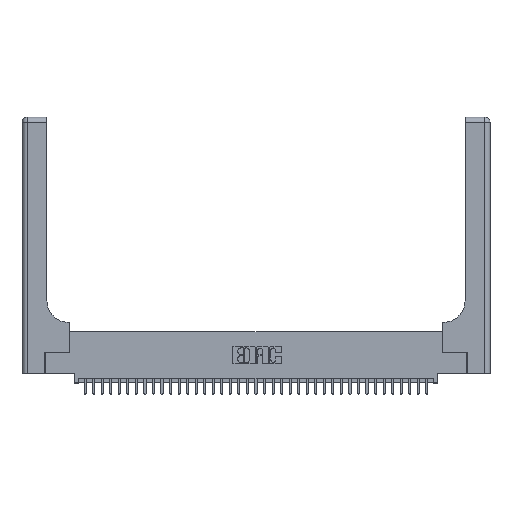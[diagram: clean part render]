
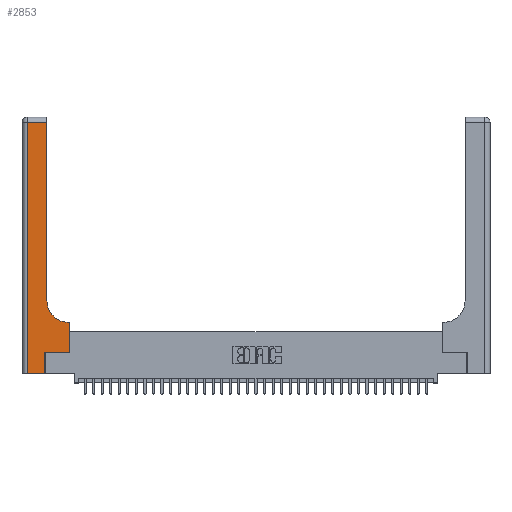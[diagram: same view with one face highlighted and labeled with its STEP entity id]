
A CAD part, top view. The second image highlights one B-rep face of the part: STEP entity #2853.
In plain terms, the highlighted planar face has unit normal (0, 0, 1).
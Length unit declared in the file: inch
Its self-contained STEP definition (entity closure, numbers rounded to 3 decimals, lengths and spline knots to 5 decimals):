
#905 = CARTESIAN_POINT ( 'NONE',  ( 0.269, 0., 0.37 ) ) ;
#2795 = VECTOR ( 'NONE', #10606, 39.37008 ) ;
#2853 = ADVANCED_FACE ( 'NONE', ( #34751 ), #29585, .F. ) ;
#3698 = VECTOR ( 'NONE', #23925, 39.37008 ) ;
#4071 = EDGE_CURVE ( 'NONE', #8317, #31394, #30599, .T. ) ;
#4381 = CARTESIAN_POINT ( 'NONE',  ( 0.269, 0.25, 0.37 ) ) ;
#4524 = DIRECTION ( 'NONE',  ( 1., 0., 0. ) ) ;
#4832 = CARTESIAN_POINT ( 'NONE',  ( 0.2915, 0.6, 0.37 ) ) ;
#5207 = DIRECTION ( 'NONE',  ( -1., 0., 0. ) ) ;
#5874 = EDGE_CURVE ( 'NONE', #9126, #23208, #30450, .T. ) ;
#6707 = ORIENTED_EDGE ( 'NONE', *, *, #24233, .T. ) ;
#7467 = VERTEX_POINT ( 'NONE', #4381 ) ;
#8197 = CARTESIAN_POINT ( 'NONE',  ( 0.2915, 2.94, 0.37 ) ) ;
#8317 = VERTEX_POINT ( 'NONE', #22243 ) ;
#9126 = VERTEX_POINT ( 'NONE', #8197 ) ;
#9229 = CARTESIAN_POINT ( 'NONE',  ( 0.269, 0., 0.37 ) ) ;
#10606 = DIRECTION ( 'NONE',  ( 0., 1., 0. ) ) ;
#10886 = CARTESIAN_POINT ( 'NONE',  ( 0.5415, 0.85, 0.37 ) ) ;
#11443 = VERTEX_POINT ( 'NONE', #30792 ) ;
#11769 = DIRECTION ( 'NONE',  ( 0., 0., -1. ) ) ;
#12270 = CARTESIAN_POINT ( 'NONE',  ( 0., 3., 0.37 ) ) ;
#12569 = ORIENTED_EDGE ( 'NONE', *, *, #26493, .T. ) ;
#13394 = CARTESIAN_POINT ( 'NONE',  ( 0.5585, 0.25, 0.37 ) ) ;
#13497 = EDGE_CURVE ( 'NONE', #31394, #7467, #32651, .T. ) ;
#14502 = DIRECTION ( 'NONE',  ( 0., -1., 0. ) ) ;
#15066 = DIRECTION ( 'NONE',  ( 0., 1., 0. ) ) ;
#16589 = LINE ( 'NONE', #25173, #21145 ) ;
#17792 = VERTEX_POINT ( 'NONE', #24611 ) ;
#18271 = EDGE_CURVE ( 'NONE', #7467, #28754, #29657, .T. ) ;
#18658 = EDGE_LOOP ( 'NONE', ( #36501, #22515, #12569, #22417, #20735, #31339, #27464, #6707, #30149 ) ) ;
#20735 = ORIENTED_EDGE ( 'NONE', *, *, #13497, .T. ) ;
#21145 = VECTOR ( 'NONE', #30897, 39.37008 ) ;
#21361 = CARTESIAN_POINT ( 'NONE',  ( 0.269, 0.25, 0.37 ) ) ;
#22243 = CARTESIAN_POINT ( 'NONE',  ( 0.06, 0., 0.37 ) ) ;
#22417 = ORIENTED_EDGE ( 'NONE', *, *, #4071, .T. ) ;
#22515 = ORIENTED_EDGE ( 'NONE', *, *, #5874, .T. ) ;
#23208 = VERTEX_POINT ( 'NONE', #29450 ) ;
#23925 = DIRECTION ( 'NONE',  ( 1., 0., 0. ) ) ;
#24233 = EDGE_CURVE ( 'NONE', #17792, #11443, #32466, .T. ) ;
#24611 = CARTESIAN_POINT ( 'NONE',  ( 0.5585, 0.6, 0.37 ) ) ;
#24971 = VECTOR ( 'NONE', #35437, 39.37008 ) ;
#25109 = AXIS2_PLACEMENT_3D ( 'NONE', #12270, #11769, #26641 ) ;
#25173 = CARTESIAN_POINT ( 'NONE',  ( 0.2915, 3., 0.37 ) ) ;
#25206 = CARTESIAN_POINT ( 'NONE',  ( 0.5585, 0.25, 0.37 ) ) ;
#25261 = EDGE_CURVE ( 'NONE', #28754, #17792, #32436, .T. ) ;
#26493 = EDGE_CURVE ( 'NONE', #23208, #8317, #37329, .T. ) ;
#26641 = DIRECTION ( 'NONE',  ( -1., 0., 0. ) ) ;
#27053 = VERTEX_POINT ( 'NONE', #28631 ) ;
#27394 = EDGE_CURVE ( 'NONE', #27053, #9126, #16589, .T. ) ;
#27464 = ORIENTED_EDGE ( 'NONE', *, *, #25261, .T. ) ;
#28631 = CARTESIAN_POINT ( 'NONE',  ( 0.2915, 0.85, 0.37 ) ) ;
#28754 = VERTEX_POINT ( 'NONE', #25206 ) ;
#29450 = CARTESIAN_POINT ( 'NONE',  ( 0.06, 2.94, 0.37 ) ) ;
#29585 = PLANE ( 'NONE',  #25109 ) ;
#29657 = LINE ( 'NONE', #21361, #3698 ) ;
#29946 = VECTOR ( 'NONE', #15066, 39.37008 ) ;
#29999 = CARTESIAN_POINT ( 'NONE',  ( 0., 2.94, 0.37 ) ) ;
#30149 = ORIENTED_EDGE ( 'NONE', *, *, #33298, .T. ) ;
#30450 = LINE ( 'NONE', #29999, #24971 ) ;
#30599 = LINE ( 'NONE', #35593, #31072 ) ;
#30777 = CIRCLE ( 'NONE', #31542, 0.25 ) ;
#30792 = CARTESIAN_POINT ( 'NONE',  ( 0.5415, 0.6, 0.37 ) ) ;
#30897 = DIRECTION ( 'NONE',  ( 0., 1., 0. ) ) ;
#31072 = VECTOR ( 'NONE', #35463, 39.37008 ) ;
#31339 = ORIENTED_EDGE ( 'NONE', *, *, #18271, .T. ) ;
#31394 = VERTEX_POINT ( 'NONE', #905 ) ;
#31542 = AXIS2_PLACEMENT_3D ( 'NONE', #10886, #34146, #4524 ) ;
#31546 = VECTOR ( 'NONE', #5207, 39.37008 ) ;
#32436 = LINE ( 'NONE', #13394, #2795 ) ;
#32466 = LINE ( 'NONE', #4832, #31546 ) ;
#32651 = LINE ( 'NONE', #9229, #29946 ) ;
#33298 = EDGE_CURVE ( 'NONE', #11443, #27053, #30777, .T. ) ;
#34146 = DIRECTION ( 'NONE',  ( 0., 0., -1. ) ) ;
#34728 = CARTESIAN_POINT ( 'NONE',  ( 0.06, 3., 0.37 ) ) ;
#34751 = FACE_OUTER_BOUND ( 'NONE', #18658, .T. ) ;
#35437 = DIRECTION ( 'NONE',  ( -1., 0., 0. ) ) ;
#35463 = DIRECTION ( 'NONE',  ( 1., 0., 0. ) ) ;
#35593 = CARTESIAN_POINT ( 'NONE',  ( 0., 0., 0.37 ) ) ;
#36501 = ORIENTED_EDGE ( 'NONE', *, *, #27394, .T. ) ;
#36860 = VECTOR ( 'NONE', #14502, 39.37008 ) ;
#37329 = LINE ( 'NONE', #34728, #36860 ) ;
